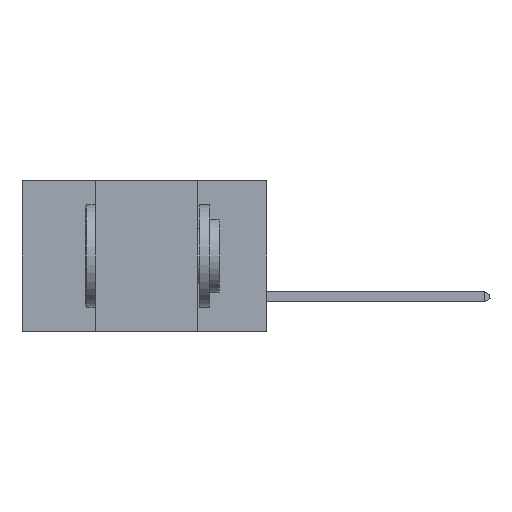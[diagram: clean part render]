
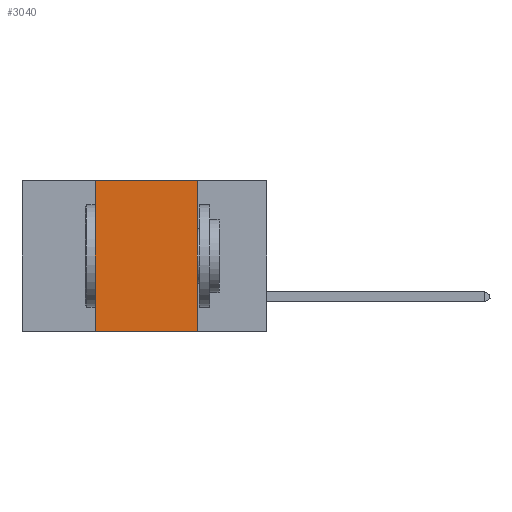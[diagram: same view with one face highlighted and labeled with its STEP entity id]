
A CAD part, left-side view. The second image highlights one B-rep face of the part: STEP entity #3040.
In plain terms, the highlighted planar face has unit normal (-1, 0, 0).
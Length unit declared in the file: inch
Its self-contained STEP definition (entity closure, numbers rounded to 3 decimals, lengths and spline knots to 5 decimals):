
#1104 = DIRECTION ( 'NONE',  ( 1., 0., 0. ) ) ;
#3040 = ADVANCED_FACE ( 'NONE', ( #24730 ), #25431, .F. ) ;
#4282 = EDGE_CURVE ( 'NONE', #27366, #8122, #22549, .T. ) ;
#4559 = EDGE_CURVE ( 'NONE', #24080, #22399, #12885, .T. ) ;
#6490 = CARTESIAN_POINT ( 'NONE',  ( 0., 0.42, -0.37 ) ) ;
#7037 = ORIENTED_EDGE ( 'NONE', *, *, #4282, .T. ) ;
#8049 = CARTESIAN_POINT ( 'NONE',  ( 0., 0.6, -0.37 ) ) ;
#8122 = VERTEX_POINT ( 'NONE', #17913 ) ;
#8731 = LINE ( 'NONE', #16879, #21898 ) ;
#9400 = DIRECTION ( 'NONE',  ( 0., -1., 0. ) ) ;
#9742 = EDGE_LOOP ( 'NONE', ( #13979, #10578, #17963, #7037 ) ) ;
#10578 = ORIENTED_EDGE ( 'NONE', *, *, #4559, .F. ) ;
#12693 = DIRECTION ( 'NONE',  ( 0., 0., -1. ) ) ;
#12885 = LINE ( 'NONE', #14067, #26340 ) ;
#13026 = DIRECTION ( 'NONE',  ( 0., 0., 1. ) ) ;
#13979 = ORIENTED_EDGE ( 'NONE', *, *, #14874, .F. ) ;
#14067 = CARTESIAN_POINT ( 'NONE',  ( 0., 0.6, 0. ) ) ;
#14434 = CARTESIAN_POINT ( 'NONE',  ( 0., 0.6, 0. ) ) ;
#14565 = DIRECTION ( 'NONE',  ( 0., -1., 0. ) ) ;
#14874 = EDGE_CURVE ( 'NONE', #22399, #8122, #25539, .T. ) ;
#15991 = VECTOR ( 'NONE', #14565, 39.37008 ) ;
#16879 = CARTESIAN_POINT ( 'NONE',  ( 0., 0.42, 0. ) ) ;
#16918 = CARTESIAN_POINT ( 'NONE',  ( 0., 0.17, 0. ) ) ;
#17913 = CARTESIAN_POINT ( 'NONE',  ( 0., 0.17, -0.37 ) ) ;
#17963 = ORIENTED_EDGE ( 'NONE', *, *, #23119, .F. ) ;
#18070 = AXIS2_PLACEMENT_3D ( 'NONE', #14434, #1104, #12693 ) ;
#18238 = VECTOR ( 'NONE', #25809, 39.37008 ) ;
#21898 = VECTOR ( 'NONE', #13026, 39.37008 ) ;
#22399 = VERTEX_POINT ( 'NONE', #16918 ) ;
#22549 = LINE ( 'NONE', #8049, #15991 ) ;
#23119 = EDGE_CURVE ( 'NONE', #27366, #24080, #8731, .T. ) ;
#23578 = CARTESIAN_POINT ( 'NONE',  ( 0., 0.17, 0. ) ) ;
#24080 = VERTEX_POINT ( 'NONE', #24366 ) ;
#24366 = CARTESIAN_POINT ( 'NONE',  ( 0., 0.42, 0. ) ) ;
#24730 = FACE_OUTER_BOUND ( 'NONE', #9742, .T. ) ;
#25431 = PLANE ( 'NONE',  #18070 ) ;
#25539 = LINE ( 'NONE', #23578, #18238 ) ;
#25809 = DIRECTION ( 'NONE',  ( 0., 0., -1. ) ) ;
#26340 = VECTOR ( 'NONE', #9400, 39.37008 ) ;
#27366 = VERTEX_POINT ( 'NONE', #6490 ) ;
